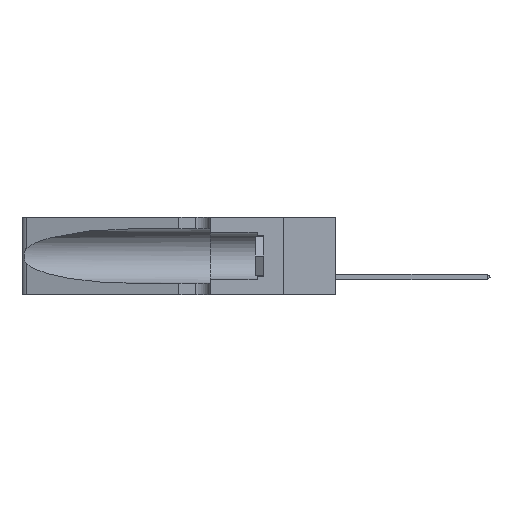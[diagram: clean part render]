
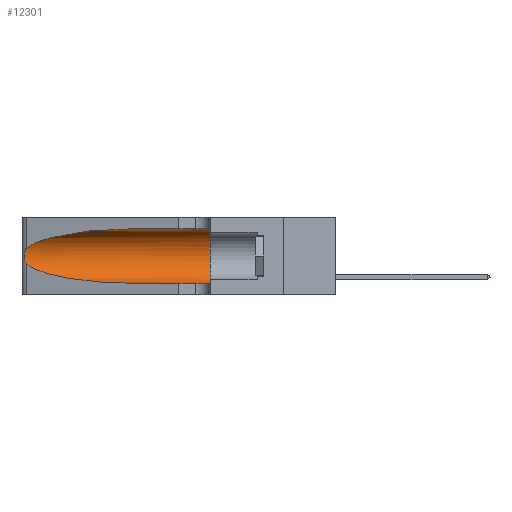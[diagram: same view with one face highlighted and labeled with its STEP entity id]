
A CAD part, left-side view. The second image highlights one B-rep face of the part: STEP entity #12301.
In plain terms, the highlighted cylindrical face has radius 3.308 mm (diameter 6.617 mm), a partial arc.
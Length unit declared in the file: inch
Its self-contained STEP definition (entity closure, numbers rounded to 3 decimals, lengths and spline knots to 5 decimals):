
#55 = EDGE_CURVE ( 'NONE', #10502, #7915, #24539, .T. ) ;
#203 = ORIENTED_EDGE ( 'NONE', *, *, #15752, .T. ) ;
#1480 = CARTESIAN_POINT ( 'NONE',  ( 0.1305, 0.72297, 0.05475 ) ) ;
#1635 = CARTESIAN_POINT ( 'NONE',  ( 0.1305, 1.61858, 0.05475 ) ) ;
#2134 = EDGE_CURVE ( 'NONE', #7915, #13209, #19826, .T. ) ;
#3063 = LINE ( 'NONE', #1635, #23535 ) ;
#3218 = CARTESIAN_POINT ( 'NONE',  ( 0.25487, 1.22718, 0.14631 ) ) ;
#3340 = CARTESIAN_POINT ( 'NONE',  ( 0.25854, 1.2359, 0.20912 ) ) ;
#3716 = DIRECTION ( 'NONE',  ( 0., 1., 0. ) ) ;
#4364 = CARTESIAN_POINT ( 'NONE',  ( 0.18966, 0.96281, 0.31525 ) ) ;
#4775 =( BOUNDED_CURVE ( )  B_SPLINE_CURVE ( 3, ( #3218, #7059, #10873, #16579 ),
 .UNSPECIFIED., .F., .F. ) 
 B_SPLINE_CURVE_WITH_KNOTS ( ( 4, 4 ),
 ( 3.44316, 4.71239 ),
 .UNSPECIFIED. ) 
 CURVE ( )  GEOMETRIC_REPRESENTATION_ITEM ( )  RATIONAL_B_SPLINE_CURVE ( ( 1., 0.87, 0.87, 1. ) ) 
 REPRESENTATION_ITEM ( '' )  );
#5261 = CARTESIAN_POINT ( 'NONE',  ( 0.26018, 1.23835, 0.19895 ) ) ;
#5342 = CARTESIAN_POINT ( 'NONE',  ( 0.25639, 1.23186, 0.15144 ) ) ;
#5426 = CARTESIAN_POINT ( 'NONE',  ( 0.26075, 1.23896, 0.19203 ) ) ;
#6287 = CARTESIAN_POINT ( 'NONE',  ( 0.2373, 1.15595, 0.28018 ) ) ;
#7015 = CARTESIAN_POINT ( 'NONE',  ( 0.25856, 1.23593, 0.16098 ) ) ;
#7059 = CARTESIAN_POINT ( 'NONE',  ( 0.2373, 1.15595, 0.08982 ) ) ;
#7157 = CARTESIAN_POINT ( 'NONE',  ( 0.1305, 0.35, 0.31525 ) ) ;
#7270 = CARTESIAN_POINT ( 'NONE',  ( 0.25789, 1.23486, 0.15765 ) ) ;
#7810 = FACE_OUTER_BOUND ( 'NONE', #12212, .T. ) ;
#7915 = VERTEX_POINT ( 'NONE', #20755 ) ;
#8122 = DIRECTION ( 'NONE',  ( 0., -1., 0. ) ) ;
#8579 = CARTESIAN_POINT ( 'NONE',  ( 0.1305, 0.72297, 0.31525 ) ) ;
#8935 = CARTESIAN_POINT ( 'NONE',  ( 0.25487, 1.22718, 0.14631 ) ) ;
#8959 = CIRCLE ( 'NONE', #17018, 0.13025 ) ;
#9003 = DIRECTION ( 'NONE',  ( 0., -1., 0. ) ) ;
#9561 = ORIENTED_EDGE ( 'NONE', *, *, #55, .T. ) ;
#9947 = ORIENTED_EDGE ( 'NONE', *, *, #17389, .F. ) ;
#10502 = VERTEX_POINT ( 'NONE', #8579 ) ;
#10873 = CARTESIAN_POINT ( 'NONE',  ( 0.18966, 0.96281, 0.05475 ) ) ;
#11898 = CARTESIAN_POINT ( 'NONE',  ( 0.1305, 0.72297, 0.31525 ) ) ;
#12212 = EDGE_LOOP ( 'NONE', ( #9561, #16359, #21251, #203, #18117, #9947 ) ) ;
#12301 = ADVANCED_FACE ( 'NONE', ( #7810 ), #16982, .F. ) ;
#12497 = VERTEX_POINT ( 'NONE', #1480 ) ;
#12555 = CARTESIAN_POINT ( 'NONE',  ( 0.25487, 1.22718, 0.22369 ) ) ;
#12905 = CARTESIAN_POINT ( 'NONE',  ( 0.1305, 0.35, 0.05475 ) ) ;
#12948 = EDGE_CURVE ( 'NONE', #24290, #23842, #8959, .T. ) ;
#12979 = CARTESIAN_POINT ( 'NONE',  ( 0.25487, 1.22718, 0.22369 ) ) ;
#13209 = VERTEX_POINT ( 'NONE', #20176 ) ;
#14782 = CARTESIAN_POINT ( 'NONE',  ( 0.25639, 1.23184, 0.21858 ) ) ;
#14886 = DIRECTION ( 'NONE',  ( 0., -1., 0. ) ) ;
#15153 = DIRECTION ( 'NONE',  ( 0., 0., 1. ) ) ;
#15752 = EDGE_CURVE ( 'NONE', #12497, #23842, #3063, .T. ) ;
#16359 = ORIENTED_EDGE ( 'NONE', *, *, #2134, .T. ) ;
#16579 = CARTESIAN_POINT ( 'NONE',  ( 0.1305, 0.72297, 0.05475 ) ) ;
#16705 = CARTESIAN_POINT ( 'NONE',  ( 0.26017, 1.23833, 0.17102 ) ) ;
#16787 = CARTESIAN_POINT ( 'NONE',  ( 0.25787, 1.23484, 0.2124 ) ) ;
#16982 = CYLINDRICAL_SURFACE ( 'NONE', #19091, 0.13025 ) ;
#17018 = AXIS2_PLACEMENT_3D ( 'NONE', #18974, #3716, #15153 ) ;
#17244 = LINE ( 'NONE', #22307, #18734 ) ;
#17389 = EDGE_CURVE ( 'NONE', #10502, #24290, #17244, .T. ) ;
#17483 = DIRECTION ( 'NONE',  ( 0., 0., -1. ) ) ;
#18117 = ORIENTED_EDGE ( 'NONE', *, *, #12948, .F. ) ;
#18621 = CARTESIAN_POINT ( 'NONE',  ( 0.25555, 1.22993, 0.14849 ) ) ;
#18734 = VECTOR ( 'NONE', #9003, 39.37008 ) ;
#18974 = CARTESIAN_POINT ( 'NONE',  ( 0.1305, 0.35, 0.185 ) ) ;
#19091 = AXIS2_PLACEMENT_3D ( 'NONE', #19623, #8122, #17483 ) ;
#19623 = CARTESIAN_POINT ( 'NONE',  ( 0.1305, 1.61858, 0.185 ) ) ;
#19826 = B_SPLINE_CURVE_WITH_KNOTS ( 'NONE', 3,
 ( #12979, #24289, #14782, #16787, #3340, #5261, #5426, #20264, #16705, #7015, #7270, #5342, #18621, #8935 ),
 .UNSPECIFIED., .F., .F.,
 ( 4, 2, 2, 2, 2, 2, 4 ),
 ( 0., 0.00027, 0.00053, 0.00107, 0.0016, 0.00187, 0.00214 ),
 .UNSPECIFIED. ) ;
#20176 = CARTESIAN_POINT ( 'NONE',  ( 0.25487, 1.22718, 0.14631 ) ) ;
#20264 = CARTESIAN_POINT ( 'NONE',  ( 0.26075, 1.23896, 0.178 ) ) ;
#20755 = CARTESIAN_POINT ( 'NONE',  ( 0.25487, 1.22718, 0.22369 ) ) ;
#21233 = EDGE_CURVE ( 'NONE', #13209, #12497, #4775, .T. ) ;
#21251 = ORIENTED_EDGE ( 'NONE', *, *, #21233, .T. ) ;
#22307 = CARTESIAN_POINT ( 'NONE',  ( 0.1305, 1.61858, 0.31525 ) ) ;
#23535 = VECTOR ( 'NONE', #14886, 39.37008 ) ;
#23842 = VERTEX_POINT ( 'NONE', #12905 ) ;
#24289 = CARTESIAN_POINT ( 'NONE',  ( 0.25555, 1.22994, 0.2215 ) ) ;
#24290 = VERTEX_POINT ( 'NONE', #7157 ) ;
#24539 =( BOUNDED_CURVE ( )  B_SPLINE_CURVE ( 3, ( #11898, #4364, #6287, #12555 ),
 .UNSPECIFIED., .F., .F. ) 
 B_SPLINE_CURVE_WITH_KNOTS ( ( 4, 4 ),
 ( 1.5708, 2.84003 ),
 .UNSPECIFIED. ) 
 CURVE ( )  GEOMETRIC_REPRESENTATION_ITEM ( )  RATIONAL_B_SPLINE_CURVE ( ( 1., 0.87, 0.87, 1. ) ) 
 REPRESENTATION_ITEM ( '' )  );
